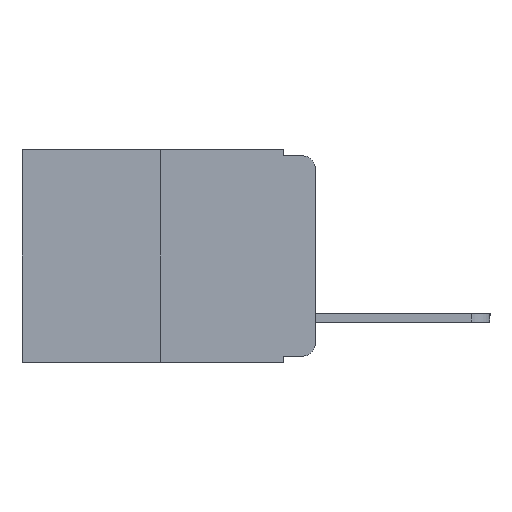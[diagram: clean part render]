
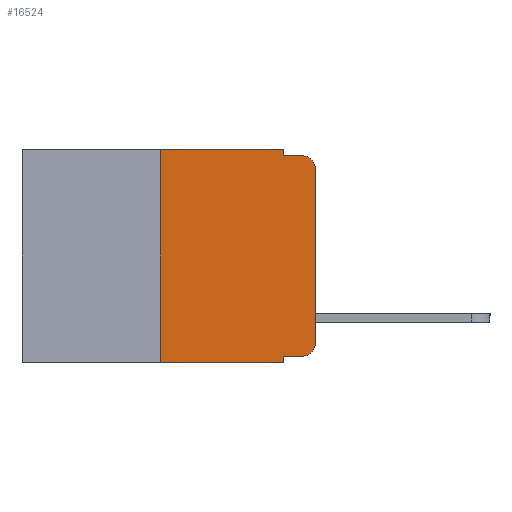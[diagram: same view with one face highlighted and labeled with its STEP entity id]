
A CAD part, left-side view. The second image highlights one B-rep face of the part: STEP entity #16524.
In plain terms, the highlighted planar face has unit normal (-1, 0, 0).
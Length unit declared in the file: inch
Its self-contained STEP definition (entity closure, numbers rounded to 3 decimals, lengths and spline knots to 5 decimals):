
#39 = LINE ( 'NONE', #9803, #20213 ) ;
#48 = VECTOR ( 'NONE', #8186, 39.37008 ) ;
#157 = VERTEX_POINT ( 'NONE', #20933 ) ;
#346 = VECTOR ( 'NONE', #4850, 39.37008 ) ;
#600 = DIRECTION ( 'NONE',  ( 0., -1., 0. ) ) ;
#720 = DIRECTION ( 'NONE',  ( 0., 0., -1. ) ) ;
#888 = CARTESIAN_POINT ( 'NONE',  ( 0., 0.25, 0. ) ) ;
#938 = EDGE_CURVE ( 'NONE', #20165, #8804, #39, .T. ) ;
#991 = DIRECTION ( 'NONE',  ( 0., 0., -1. ) ) ;
#1179 = CARTESIAN_POINT ( 'NONE',  ( 0., 0., -0.03 ) ) ;
#1667 = DIRECTION ( 'NONE',  ( 0., 0., 1. ) ) ;
#1794 = VERTEX_POINT ( 'NONE', #8031 ) ;
#1804 = EDGE_CURVE ( 'NONE', #22951, #157, #15683, .T. ) ;
#1834 = CARTESIAN_POINT ( 'NONE',  ( 0., 0.473, 0. ) ) ;
#2428 = VECTOR ( 'NONE', #15920, 39.37008 ) ;
#2619 = CARTESIAN_POINT ( 'NONE',  ( 0., 0., 0. ) ) ;
#3266 = VECTOR ( 'NONE', #7662, 39.37008 ) ;
#3877 = DIRECTION ( 'NONE',  ( 0., 0., -1. ) ) ;
#4422 = LINE ( 'NONE', #22100, #19333 ) ;
#4850 = DIRECTION ( 'NONE',  ( 0., 0., 1. ) ) ;
#5675 = LINE ( 'NONE', #888, #346 ) ;
#6233 = CARTESIAN_POINT ( 'NONE',  ( 0., 0.051, 0. ) ) ;
#6740 = EDGE_LOOP ( 'NONE', ( #16796, #9322, #16859, #16351, #14216, #23130, #22017, #14354, #7445, #14795 ) ) ;
#6835 = EDGE_CURVE ( 'NONE', #157, #8436, #18852, .T. ) ;
#7062 = DIRECTION ( 'NONE',  ( 0., -1., 0. ) ) ;
#7313 = VERTEX_POINT ( 'NONE', #9408 ) ;
#7379 = AXIS2_PLACEMENT_3D ( 'NONE', #12999, #7519, #991 ) ;
#7416 = AXIS2_PLACEMENT_3D ( 'NONE', #1834, #15573, #3877 ) ;
#7426 = CARTESIAN_POINT ( 'NONE',  ( 0., 0.051, -0.333 ) ) ;
#7445 = ORIENTED_EDGE ( 'NONE', *, *, #16772, .T. ) ;
#7519 = DIRECTION ( 'NONE',  ( -1., 0., 0. ) ) ;
#7554 = CARTESIAN_POINT ( 'NONE',  ( 0., 0.02, -0.03 ) ) ;
#7662 = DIRECTION ( 'NONE',  ( 0., -1., 0. ) ) ;
#7745 = LINE ( 'NONE', #6233, #2428 ) ;
#7920 = CARTESIAN_POINT ( 'NONE',  ( 0., 0.25, -0.343 ) ) ;
#8031 = CARTESIAN_POINT ( 'NONE',  ( 0., 0.02, -0.01 ) ) ;
#8186 = DIRECTION ( 'NONE',  ( 0., -1., 0. ) ) ;
#8324 = CARTESIAN_POINT ( 'NONE',  ( 0., 0.051, 0. ) ) ;
#8343 = CARTESIAN_POINT ( 'NONE',  ( 0., 0.02, -0.333 ) ) ;
#8436 = VERTEX_POINT ( 'NONE', #1179 ) ;
#8555 = VECTOR ( 'NONE', #1667, 39.37008 ) ;
#8692 = CIRCLE ( 'NONE', #23008, 0.02 ) ;
#8804 = VERTEX_POINT ( 'NONE', #8324 ) ;
#8960 = EDGE_CURVE ( 'NONE', #15457, #20165, #5675, .T. ) ;
#9255 = LINE ( 'NONE', #12423, #24544 ) ;
#9322 = ORIENTED_EDGE ( 'NONE', *, *, #15956, .T. ) ;
#9408 = CARTESIAN_POINT ( 'NONE',  ( 0., 0.051, -0.01 ) ) ;
#9498 = DIRECTION ( 'NONE',  ( 0., 0., -1. ) ) ;
#9803 = CARTESIAN_POINT ( 'NONE',  ( 0., 0.473, 0. ) ) ;
#10382 = CARTESIAN_POINT ( 'NONE',  ( 0., 0.051, -0.343 ) ) ;
#10597 = LINE ( 'NONE', #21655, #48 ) ;
#11576 = EDGE_CURVE ( 'NONE', #19678, #24204, #4422, .T. ) ;
#12423 = CARTESIAN_POINT ( 'NONE',  ( 0., 0.051, -0.333 ) ) ;
#12999 = CARTESIAN_POINT ( 'NONE',  ( 0., 0.02, -0.313 ) ) ;
#13704 = LINE ( 'NONE', #21144, #3266 ) ;
#14110 = FACE_OUTER_BOUND ( 'NONE', #6740, .T. ) ;
#14216 = ORIENTED_EDGE ( 'NONE', *, *, #938, .F. ) ;
#14354 = ORIENTED_EDGE ( 'NONE', *, *, #11576, .F. ) ;
#14795 = ORIENTED_EDGE ( 'NONE', *, *, #1804, .T. ) ;
#15457 = VERTEX_POINT ( 'NONE', #7920 ) ;
#15573 = DIRECTION ( 'NONE',  ( 1., 0., 0. ) ) ;
#15683 = CIRCLE ( 'NONE', #7379, 0.02 ) ;
#15920 = DIRECTION ( 'NONE',  ( 0., 0., -1. ) ) ;
#15956 = EDGE_CURVE ( 'NONE', #8436, #1794, #8692, .T. ) ;
#16351 = ORIENTED_EDGE ( 'NONE', *, *, #22322, .F. ) ;
#16524 = ADVANCED_FACE ( 'NONE', ( #14110 ), #25046, .F. ) ;
#16772 = EDGE_CURVE ( 'NONE', #19678, #22951, #9255, .T. ) ;
#16796 = ORIENTED_EDGE ( 'NONE', *, *, #6835, .T. ) ;
#16859 = ORIENTED_EDGE ( 'NONE', *, *, #18518, .F. ) ;
#18518 = EDGE_CURVE ( 'NONE', #7313, #1794, #13704, .T. ) ;
#18852 = LINE ( 'NONE', #2619, #8555 ) ;
#19333 = VECTOR ( 'NONE', #720, 39.37008 ) ;
#19678 = VERTEX_POINT ( 'NONE', #7426 ) ;
#20165 = VERTEX_POINT ( 'NONE', #24260 ) ;
#20213 = VECTOR ( 'NONE', #7062, 39.37008 ) ;
#20933 = CARTESIAN_POINT ( 'NONE',  ( 0., 0., -0.313 ) ) ;
#21041 = DIRECTION ( 'NONE',  ( -1., 0., 0. ) ) ;
#21043 = EDGE_CURVE ( 'NONE', #15457, #24204, #10597, .T. ) ;
#21144 = CARTESIAN_POINT ( 'NONE',  ( 0., 0.051, -0.01 ) ) ;
#21655 = CARTESIAN_POINT ( 'NONE',  ( 0., 0.473, -0.343 ) ) ;
#22017 = ORIENTED_EDGE ( 'NONE', *, *, #21043, .T. ) ;
#22100 = CARTESIAN_POINT ( 'NONE',  ( 0., 0.051, 0. ) ) ;
#22322 = EDGE_CURVE ( 'NONE', #8804, #7313, #7745, .T. ) ;
#22951 = VERTEX_POINT ( 'NONE', #8343 ) ;
#23008 = AXIS2_PLACEMENT_3D ( 'NONE', #7554, #21041, #9498 ) ;
#23130 = ORIENTED_EDGE ( 'NONE', *, *, #8960, .F. ) ;
#24204 = VERTEX_POINT ( 'NONE', #10382 ) ;
#24260 = CARTESIAN_POINT ( 'NONE',  ( 0., 0.25, 0. ) ) ;
#24544 = VECTOR ( 'NONE', #600, 39.37008 ) ;
#25046 = PLANE ( 'NONE',  #7416 ) ;
